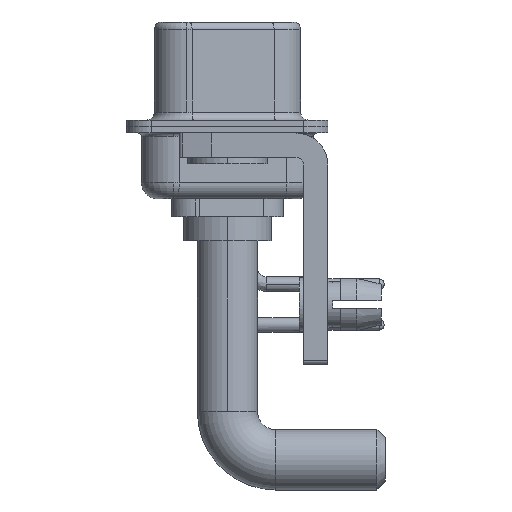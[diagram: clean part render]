
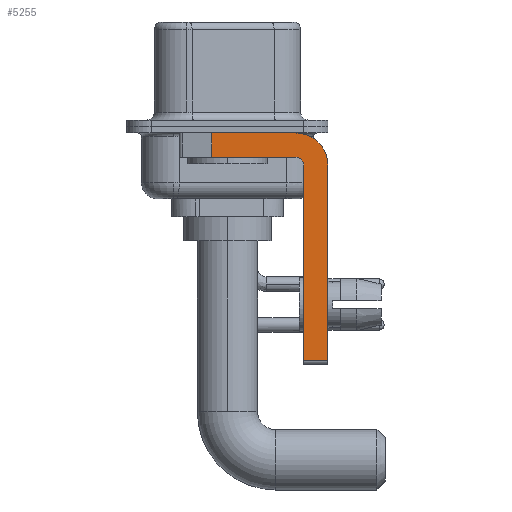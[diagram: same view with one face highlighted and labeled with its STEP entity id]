
A CAD part, left-side view. The second image highlights one B-rep face of the part: STEP entity #5255.
In plain terms, the highlighted planar face has unit normal (-1, 0, 0).
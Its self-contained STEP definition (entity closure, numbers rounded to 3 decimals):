
#212 = CARTESIAN_POINT ( 'NONE',  ( -2.9, -4.25, -1.9 ) ) ;
#353 = LINE ( 'NONE', #6182, #19316 ) ;
#548 = ORIENTED_EDGE ( 'NONE', *, *, #1388, .F. ) ;
#671 = VECTOR ( 'NONE', #15376, 1000. ) ;
#1388 = EDGE_CURVE ( 'NONE', #22402, #5312, #12584, .T. ) ;
#2126 = VERTEX_POINT ( 'NONE', #13888 ) ;
#2406 = CARTESIAN_POINT ( 'NONE',  ( -2.9, -4.75, -14.8 ) ) ;
#3239 = VERTEX_POINT ( 'NONE', #4110 ) ;
#3444 = DIRECTION ( 'NONE',  ( 0., 0., -1. ) ) ;
#4110 = CARTESIAN_POINT ( 'NONE',  ( -2.9, 0.978, -1.9 ) ) ;
#4145 = ORIENTED_EDGE ( 'NONE', *, *, #25344, .F. ) ;
#4343 = VECTOR ( 'NONE', #26721, 1000. ) ;
#5138 = CARTESIAN_POINT ( 'NONE',  ( -2.9, -4.75, -2.4 ) ) ;
#5255 = ADVANCED_FACE ( 'NONE', ( #8822 ), #17107, .F. ) ;
#5312 = VERTEX_POINT ( 'NONE', #5138 ) ;
#5472 = CARTESIAN_POINT ( 'NONE',  ( -2.9, -4.75, -14.55 ) ) ;
#5770 = DIRECTION ( 'NONE',  ( 1., 0., 0. ) ) ;
#5951 = ORIENTED_EDGE ( 'NONE', *, *, #5973, .F. ) ;
#5973 = EDGE_CURVE ( 'NONE', #2126, #3239, #22901, .T. ) ;
#6000 = EDGE_CURVE ( 'NONE', #5312, #2126, #12155, .T. ) ;
#6182 = CARTESIAN_POINT ( 'NONE',  ( -2.9, -6.25, -2.4 ) ) ;
#6369 = VECTOR ( 'NONE', #14890, 1000. ) ;
#6406 = VERTEX_POINT ( 'NONE', #20110 ) ;
#6512 = AXIS2_PLACEMENT_3D ( 'NONE', #18812, #8489, #16234 ) ;
#6864 = EDGE_CURVE ( 'NONE', #7629, #18434, #15456, .T. ) ;
#7044 = CARTESIAN_POINT ( 'NONE',  ( -2.9, -4.25, -2.4 ) ) ;
#7629 = VERTEX_POINT ( 'NONE', #16755 ) ;
#8489 = DIRECTION ( 'NONE',  ( -1., 0., 0. ) ) ;
#8822 = FACE_OUTER_BOUND ( 'NONE', #9232, .T. ) ;
#9133 = CARTESIAN_POINT ( 'NONE',  ( -2.9, -4.25, -14.55 ) ) ;
#9232 = EDGE_LOOP ( 'NONE', ( #17689, #13843, #5951, #14135, #548, #14506, #4145, #14062 ) ) ;
#10411 = DIRECTION ( 'NONE',  ( 0., 0., -1. ) ) ;
#10793 = CARTESIAN_POINT ( 'NONE',  ( -2.9, -6.25, -2.4 ) ) ;
#10835 = AXIS2_PLACEMENT_3D ( 'NONE', #7044, #25550, #19697 ) ;
#11654 = CARTESIAN_POINT ( 'NONE',  ( -2.9, 3., -0.4 ) ) ;
#12155 = CIRCLE ( 'NONE', #6512, 0.5 ) ;
#12584 = LINE ( 'NONE', #2406, #6369 ) ;
#13462 = LINE ( 'NONE', #9133, #671 ) ;
#13843 = ORIENTED_EDGE ( 'NONE', *, *, #19811, .T. ) ;
#13888 = CARTESIAN_POINT ( 'NONE',  ( -2.9, -4.25, -1.9 ) ) ;
#14062 = ORIENTED_EDGE ( 'NONE', *, *, #25654, .F. ) ;
#14135 = ORIENTED_EDGE ( 'NONE', *, *, #6000, .F. ) ;
#14506 = ORIENTED_EDGE ( 'NONE', *, *, #22812, .T. ) ;
#14890 = DIRECTION ( 'NONE',  ( 0., 0., 1. ) ) ;
#15376 = DIRECTION ( 'NONE',  ( 0., -1., 0. ) ) ;
#15456 = LINE ( 'NONE', #11654, #18692 ) ;
#16234 = DIRECTION ( 'NONE',  ( 0., 0., 1. ) ) ;
#16755 = CARTESIAN_POINT ( 'NONE',  ( -2.9, 0.978, -0.4 ) ) ;
#17107 = PLANE ( 'NONE',  #10835 ) ;
#17689 = ORIENTED_EDGE ( 'NONE', *, *, #6864, .F. ) ;
#17704 = LINE ( 'NONE', #23985, #24932 ) ;
#18319 = VERTEX_POINT ( 'NONE', #10793 ) ;
#18434 = VERTEX_POINT ( 'NONE', #19749 ) ;
#18692 = VECTOR ( 'NONE', #19952, 1000. ) ;
#18812 = CARTESIAN_POINT ( 'NONE',  ( -2.9, -4.25, -2.4 ) ) ;
#19316 = VECTOR ( 'NONE', #21416, 1000. ) ;
#19697 = DIRECTION ( 'NONE',  ( 0., 0., -1. ) ) ;
#19749 = CARTESIAN_POINT ( 'NONE',  ( -2.9, -4.25, -0.4 ) ) ;
#19811 = EDGE_CURVE ( 'NONE', #7629, #3239, #17704, .T. ) ;
#19952 = DIRECTION ( 'NONE',  ( 0., -1., 0. ) ) ;
#20110 = CARTESIAN_POINT ( 'NONE',  ( -2.9, -6.25, -14.55 ) ) ;
#20593 = CARTESIAN_POINT ( 'NONE',  ( -2.9, -4.25, -2.4 ) ) ;
#21416 = DIRECTION ( 'NONE',  ( 0., 0., -1. ) ) ;
#21953 = CIRCLE ( 'NONE', #22819, 2. ) ;
#22402 = VERTEX_POINT ( 'NONE', #5472 ) ;
#22812 = EDGE_CURVE ( 'NONE', #22402, #6406, #13462, .T. ) ;
#22819 = AXIS2_PLACEMENT_3D ( 'NONE', #20593, #5770, #10411 ) ;
#22901 = LINE ( 'NONE', #212, #4343 ) ;
#23985 = CARTESIAN_POINT ( 'NONE',  ( -2.9, 0.978, -1.9 ) ) ;
#24932 = VECTOR ( 'NONE', #3444, 1000. ) ;
#25344 = EDGE_CURVE ( 'NONE', #18319, #6406, #353, .T. ) ;
#25550 = DIRECTION ( 'NONE',  ( 1., 0., 0. ) ) ;
#25654 = EDGE_CURVE ( 'NONE', #18434, #18319, #21953, .T. ) ;
#26721 = DIRECTION ( 'NONE',  ( 0., 1., 0. ) ) ;
